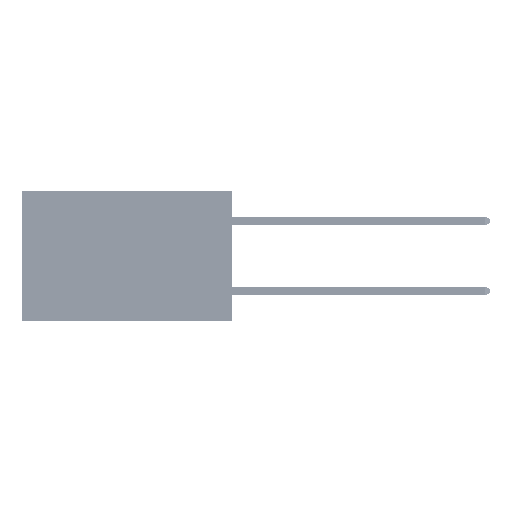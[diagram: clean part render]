
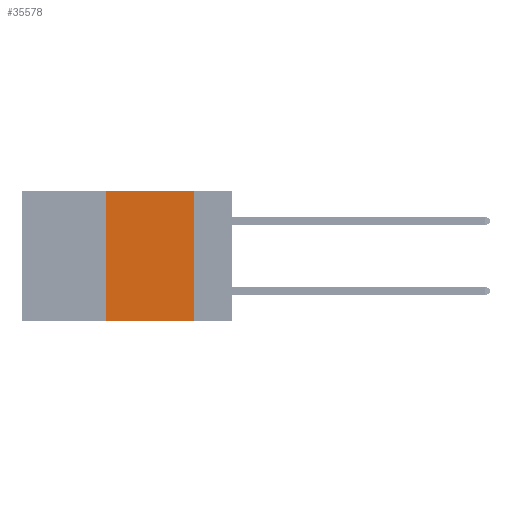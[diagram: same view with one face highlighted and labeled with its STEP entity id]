
A CAD part, left-side view. The second image highlights one B-rep face of the part: STEP entity #35578.
In plain terms, the highlighted planar face has unit normal (-1, 0, 0).
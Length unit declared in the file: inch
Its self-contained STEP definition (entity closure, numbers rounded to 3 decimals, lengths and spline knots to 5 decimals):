
#123 = EDGE_CURVE ( 'NONE', #31975, #25066, #22731, .T. ) ;
#3623 = EDGE_CURVE ( 'NONE', #31975, #38850, #44798, .T. ) ;
#5025 = CARTESIAN_POINT ( 'NONE',  ( 0., 0.36, 0. ) ) ;
#7152 = VECTOR ( 'NONE', #46548, 39.37008 ) ;
#8091 = ORIENTED_EDGE ( 'NONE', *, *, #123, .F. ) ;
#8133 = DIRECTION ( 'NONE',  ( 0., -1., 0. ) ) ;
#9324 = DIRECTION ( 'NONE',  ( 0., 0., -1. ) ) ;
#12671 = VERTEX_POINT ( 'NONE', #28754 ) ;
#12796 = VECTOR ( 'NONE', #8133, 39.37008 ) ;
#14613 = LINE ( 'NONE', #31883, #12796 ) ;
#14647 = AXIS2_PLACEMENT_3D ( 'NONE', #25625, #21322, #9324 ) ;
#16048 = ORIENTED_EDGE ( 'NONE', *, *, #48568, .F. ) ;
#21322 = DIRECTION ( 'NONE',  ( 1., 0., 0. ) ) ;
#21742 = ORIENTED_EDGE ( 'NONE', *, *, #30220, .F. ) ;
#22731 = LINE ( 'NONE', #5025, #7152 ) ;
#25066 = VERTEX_POINT ( 'NONE', #45795 ) ;
#25625 = CARTESIAN_POINT ( 'NONE',  ( 0., 0.6, 0. ) ) ;
#26275 = CARTESIAN_POINT ( 'NONE',  ( 0., 0.11, 0. ) ) ;
#26280 = VECTOR ( 'NONE', #47640, 39.37008 ) ;
#28754 = CARTESIAN_POINT ( 'NONE',  ( 0., 0.11, 0. ) ) ;
#29208 = CARTESIAN_POINT ( 'NONE',  ( 0., 0.36, -0.37 ) ) ;
#30220 = EDGE_CURVE ( 'NONE', #12671, #38850, #33932, .T. ) ;
#31883 = CARTESIAN_POINT ( 'NONE',  ( 0., 0.6, 0. ) ) ;
#31975 = VERTEX_POINT ( 'NONE', #29208 ) ;
#32943 = CARTESIAN_POINT ( 'NONE',  ( 0., 0.11, -0.37 ) ) ;
#33055 = PLANE ( 'NONE',  #14647 ) ;
#33932 = LINE ( 'NONE', #26275, #48204 ) ;
#35578 = ADVANCED_FACE ( 'NONE', ( #41312 ), #33055, .F. ) ;
#38850 = VERTEX_POINT ( 'NONE', #32943 ) ;
#41312 = FACE_OUTER_BOUND ( 'NONE', #48773, .T. ) ;
#42674 = DIRECTION ( 'NONE',  ( 0., 0., -1. ) ) ;
#43650 = CARTESIAN_POINT ( 'NONE',  ( 0., 0.6, -0.37 ) ) ;
#44798 = LINE ( 'NONE', #43650, #26280 ) ;
#45795 = CARTESIAN_POINT ( 'NONE',  ( 0., 0.36, 0. ) ) ;
#46548 = DIRECTION ( 'NONE',  ( 0., 0., 1. ) ) ;
#47640 = DIRECTION ( 'NONE',  ( 0., -1., 0. ) ) ;
#48204 = VECTOR ( 'NONE', #42674, 39.37008 ) ;
#48568 = EDGE_CURVE ( 'NONE', #25066, #12671, #14613, .T. ) ;
#48773 = EDGE_LOOP ( 'NONE', ( #21742, #16048, #8091, #50064 ) ) ;
#50064 = ORIENTED_EDGE ( 'NONE', *, *, #3623, .T. ) ;
